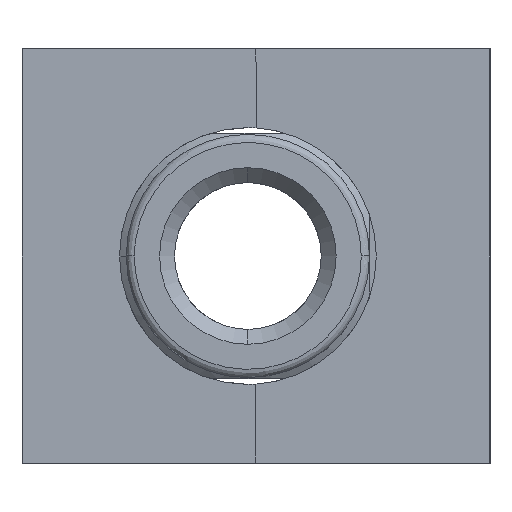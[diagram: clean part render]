
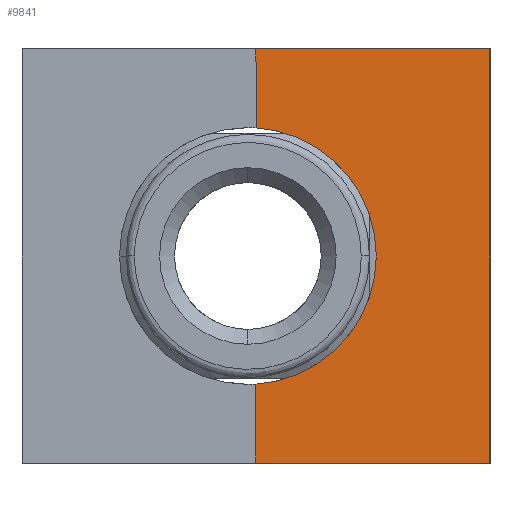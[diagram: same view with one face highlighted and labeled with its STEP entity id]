
A CAD part, left-side view. The second image highlights one B-rep face of the part: STEP entity #9841.
In plain terms, the highlighted face is planar.
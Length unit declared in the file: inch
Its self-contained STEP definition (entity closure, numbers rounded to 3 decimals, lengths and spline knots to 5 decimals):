
#39 = VERTEX_POINT ( 'NONE', #12214 ) ;
#100 = ORIENTED_EDGE ( 'NONE', *, *, #14024, .F. ) ;
#326 = VERTEX_POINT ( 'NONE', #2363 ) ;
#722 = EDGE_CURVE ( 'NONE', #6483, #326, #7883, .T. ) ;
#1532 = VERTEX_POINT ( 'NONE', #6829 ) ;
#2361 = EDGE_CURVE ( 'NONE', #39, #13549, #6271, .T. ) ;
#2363 = CARTESIAN_POINT ( 'NONE',  ( 0.19062, -0.565, 0. ) ) ;
#2605 = CARTESIAN_POINT ( 'NONE',  ( 0., -1.13, 0. ) ) ;
#3214 = DIRECTION ( 'NONE',  ( 1., 0., 0. ) ) ;
#4018 = AXIS2_PLACEMENT_3D ( 'NONE', #14712, #12520, #8713 ) ;
#4057 = ORIENTED_EDGE ( 'NONE', *, *, #5201, .T. ) ;
#4114 = DIRECTION ( 'NONE',  ( 1., 0., 0. ) ) ;
#4276 = FACE_OUTER_BOUND ( 'NONE', #7618, .T. ) ;
#5201 = EDGE_CURVE ( 'NONE', #326, #39, #5616, .T. ) ;
#5460 = CARTESIAN_POINT ( 'NONE',  ( 0., -1.13, 0. ) ) ;
#5531 = ORIENTED_EDGE ( 'NONE', *, *, #7673, .F. ) ;
#5616 = CIRCLE ( 'NONE', #4018, 0.31 ) ;
#6271 = LINE ( 'NONE', #15153, #11799 ) ;
#6417 = DIRECTION ( 'NONE',  ( 0., -1., 0. ) ) ;
#6483 = VERTEX_POINT ( 'NONE', #15436 ) ;
#6555 = CARTESIAN_POINT ( 'NONE',  ( 1., -0.565, 0. ) ) ;
#6829 = CARTESIAN_POINT ( 'NONE',  ( 1., -1.13, 0. ) ) ;
#7064 = PLANE ( 'NONE',  #12629 ) ;
#7070 = EDGE_CURVE ( 'NONE', #6483, #15485, #15144, .T. ) ;
#7343 = ORIENTED_EDGE ( 'NONE', *, *, #2361, .T. ) ;
#7618 = EDGE_LOOP ( 'NONE', ( #9334, #14071, #4057, #7343, #5531, #100 ) ) ;
#7673 = EDGE_CURVE ( 'NONE', #1532, #13549, #14478, .T. ) ;
#7883 = LINE ( 'NONE', #11789, #9987 ) ;
#8713 = DIRECTION ( 'NONE',  ( 1., 0., 0. ) ) ;
#8766 = CARTESIAN_POINT ( 'NONE',  ( 0., 0., 0. ) ) ;
#9135 = LINE ( 'NONE', #5460, #11162 ) ;
#9275 = CARTESIAN_POINT ( 'NONE',  ( 0., 0., 0. ) ) ;
#9334 = ORIENTED_EDGE ( 'NONE', *, *, #7070, .F. ) ;
#9841 = ADVANCED_FACE ( 'NONE', ( #4276 ), #7064, .F. ) ;
#9987 = VECTOR ( 'NONE', #4114, 39.37008 ) ;
#10574 = DIRECTION ( 'NONE',  ( 0., 0., 1. ) ) ;
#11162 = VECTOR ( 'NONE', #14146, 39.37008 ) ;
#11213 = DIRECTION ( 'NONE',  ( 1., 0., 0. ) ) ;
#11789 = CARTESIAN_POINT ( 'NONE',  ( 0., -0.565, 0. ) ) ;
#11799 = VECTOR ( 'NONE', #11213, 39.37008 ) ;
#12214 = CARTESIAN_POINT ( 'NONE',  ( 0.80938, -0.565, 0. ) ) ;
#12520 = DIRECTION ( 'NONE',  ( 0., 0., 1. ) ) ;
#12629 = AXIS2_PLACEMENT_3D ( 'NONE', #9275, #10574, #3214 ) ;
#13177 = CARTESIAN_POINT ( 'NONE',  ( 1., 0., 0. ) ) ;
#13549 = VERTEX_POINT ( 'NONE', #6555 ) ;
#14024 = EDGE_CURVE ( 'NONE', #15485, #1532, #9135, .T. ) ;
#14071 = ORIENTED_EDGE ( 'NONE', *, *, #722, .T. ) ;
#14146 = DIRECTION ( 'NONE',  ( 1., 0., 0. ) ) ;
#14478 = LINE ( 'NONE', #13177, #14902 ) ;
#14557 = DIRECTION ( 'NONE',  ( 0., 1., 0. ) ) ;
#14712 = CARTESIAN_POINT ( 'NONE',  ( 0.5, -0.5454, 0. ) ) ;
#14902 = VECTOR ( 'NONE', #14557, 39.37008 ) ;
#15144 = LINE ( 'NONE', #8766, #15952 ) ;
#15153 = CARTESIAN_POINT ( 'NONE',  ( 0., -0.565, 0. ) ) ;
#15436 = CARTESIAN_POINT ( 'NONE',  ( 0., -0.565, 0. ) ) ;
#15485 = VERTEX_POINT ( 'NONE', #2605 ) ;
#15952 = VECTOR ( 'NONE', #6417, 39.37008 ) ;
